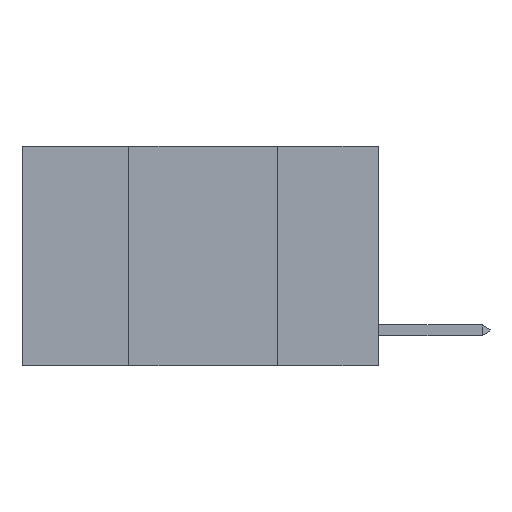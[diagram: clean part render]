
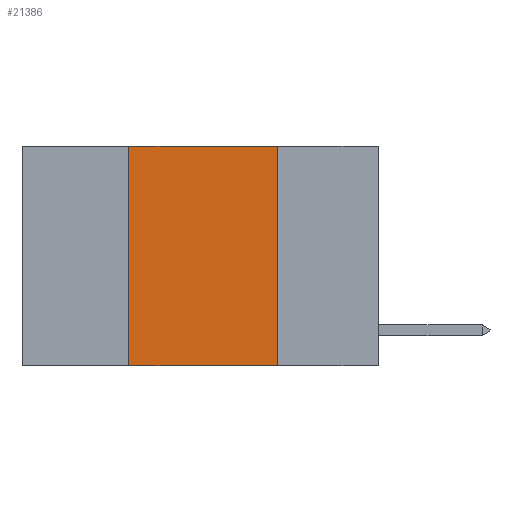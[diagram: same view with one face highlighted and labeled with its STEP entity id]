
A CAD part, left-side view. The second image highlights one B-rep face of the part: STEP entity #21386.
In plain terms, the highlighted planar face has unit normal (-1, 0, 0).
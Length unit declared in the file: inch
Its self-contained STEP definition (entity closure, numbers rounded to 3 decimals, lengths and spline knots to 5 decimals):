
#823 = VERTEX_POINT ( 'NONE', #19440 ) ;
#1109 = VECTOR ( 'NONE', #13387, 39.37008 ) ;
#1978 = AXIS2_PLACEMENT_3D ( 'NONE', #19892, #20171, #17709 ) ;
#4522 = DIRECTION ( 'NONE',  ( 0., -1., 0. ) ) ;
#4550 = ORIENTED_EDGE ( 'NONE', *, *, #8496, .F. ) ;
#4973 = LINE ( 'NONE', #26960, #21690 ) ;
#5385 = CARTESIAN_POINT ( 'NONE',  ( 0., 0.42, 0. ) ) ;
#5977 = EDGE_CURVE ( 'NONE', #8571, #7368, #22867, .T. ) ;
#7337 = CARTESIAN_POINT ( 'NONE',  ( 0., 0.17, -0.37 ) ) ;
#7368 = VERTEX_POINT ( 'NONE', #18474 ) ;
#8496 = EDGE_CURVE ( 'NONE', #7368, #823, #4973, .T. ) ;
#8571 = VERTEX_POINT ( 'NONE', #15692 ) ;
#8751 = EDGE_LOOP ( 'NONE', ( #27192, #4550, #17765, #9849 ) ) ;
#9849 = ORIENTED_EDGE ( 'NONE', *, *, #25364, .T. ) ;
#11486 = EDGE_CURVE ( 'NONE', #823, #22588, #18228, .T. ) ;
#11739 = DIRECTION ( 'NONE',  ( 0., -1., 0. ) ) ;
#13177 = CARTESIAN_POINT ( 'NONE',  ( 0., 0.6, -0.37 ) ) ;
#13387 = DIRECTION ( 'NONE',  ( 0., 0., -1. ) ) ;
#13825 = CARTESIAN_POINT ( 'NONE',  ( 0., 0.17, 0. ) ) ;
#15310 = VECTOR ( 'NONE', #25182, 39.37008 ) ;
#15692 = CARTESIAN_POINT ( 'NONE',  ( 0., 0.42, -0.37 ) ) ;
#17709 = DIRECTION ( 'NONE',  ( 0., 0., -1. ) ) ;
#17765 = ORIENTED_EDGE ( 'NONE', *, *, #5977, .F. ) ;
#18228 = LINE ( 'NONE', #13825, #1109 ) ;
#18474 = CARTESIAN_POINT ( 'NONE',  ( 0., 0.42, 0. ) ) ;
#19440 = CARTESIAN_POINT ( 'NONE',  ( 0., 0.17, 0. ) ) ;
#19892 = CARTESIAN_POINT ( 'NONE',  ( 0., 0.6, 0. ) ) ;
#20034 = PLANE ( 'NONE',  #1978 ) ;
#20171 = DIRECTION ( 'NONE',  ( 1., 0., 0. ) ) ;
#21386 = ADVANCED_FACE ( 'NONE', ( #26314 ), #20034, .F. ) ;
#21690 = VECTOR ( 'NONE', #11739, 39.37008 ) ;
#22588 = VERTEX_POINT ( 'NONE', #7337 ) ;
#22867 = LINE ( 'NONE', #5385, #15310 ) ;
#24615 = LINE ( 'NONE', #13177, #25623 ) ;
#25182 = DIRECTION ( 'NONE',  ( 0., 0., 1. ) ) ;
#25364 = EDGE_CURVE ( 'NONE', #8571, #22588, #24615, .T. ) ;
#25623 = VECTOR ( 'NONE', #4522, 39.37008 ) ;
#26314 = FACE_OUTER_BOUND ( 'NONE', #8751, .T. ) ;
#26960 = CARTESIAN_POINT ( 'NONE',  ( 0., 0.6, 0. ) ) ;
#27192 = ORIENTED_EDGE ( 'NONE', *, *, #11486, .F. ) ;
